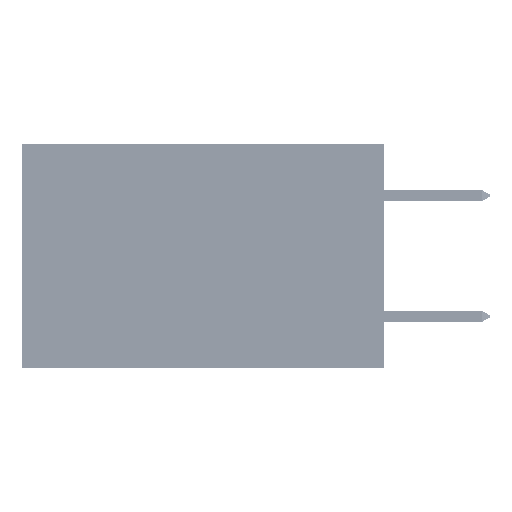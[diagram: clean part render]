
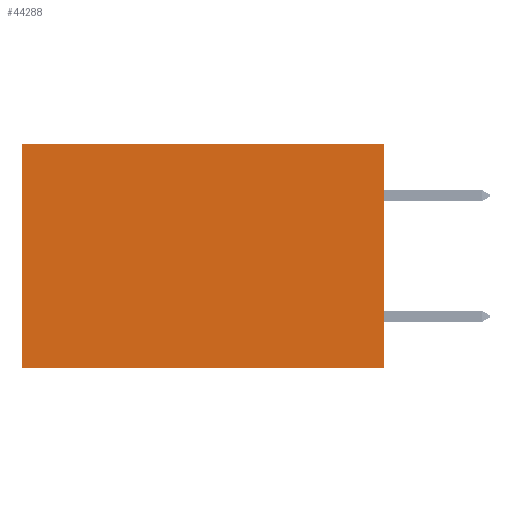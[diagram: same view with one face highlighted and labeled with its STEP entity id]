
A CAD part, left-side view. The second image highlights one B-rep face of the part: STEP entity #44288.
In plain terms, the highlighted planar face has unit normal (-1, 0, 0).
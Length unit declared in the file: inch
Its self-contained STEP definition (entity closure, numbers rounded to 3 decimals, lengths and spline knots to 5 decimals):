
#1999 = CARTESIAN_POINT ( 'NONE',  ( 0.2875, 0., 0. ) ) ;
#2432 = ORIENTED_EDGE ( 'NONE', *, *, #26261, .F. ) ;
#3375 = CARTESIAN_POINT ( 'NONE',  ( 0.2875, 0., -0.37 ) ) ;
#5676 = CARTESIAN_POINT ( 'NONE',  ( 0.2875, 0., 0. ) ) ;
#6290 = EDGE_LOOP ( 'NONE', ( #28911, #17795, #2432, #31878 ) ) ;
#8955 = CARTESIAN_POINT ( 'NONE',  ( 0.2875, 0., 0. ) ) ;
#9525 = DIRECTION ( 'NONE',  ( 0., 1., 0. ) ) ;
#9595 = PLANE ( 'NONE',  #40145 ) ;
#11863 = VECTOR ( 'NONE', #9525, 39.37008 ) ;
#17795 = ORIENTED_EDGE ( 'NONE', *, *, #31274, .F. ) ;
#17911 = DIRECTION ( 'NONE',  ( 0., 0., -1. ) ) ;
#19109 = VERTEX_POINT ( 'NONE', #43107 ) ;
#19327 = CARTESIAN_POINT ( 'NONE',  ( 0.2875, 0.6, -0.37 ) ) ;
#23286 = LINE ( 'NONE', #3375, #30376 ) ;
#25293 = DIRECTION ( 'NONE',  ( 0., 1., 0. ) ) ;
#26261 = EDGE_CURVE ( 'NONE', #33278, #19109, #46434, .T. ) ;
#26649 = DIRECTION ( 'NONE',  ( 0., 0., -1. ) ) ;
#28791 = EDGE_CURVE ( 'NONE', #33278, #43486, #31813, .T. ) ;
#28911 = ORIENTED_EDGE ( 'NONE', *, *, #46445, .T. ) ;
#30376 = VECTOR ( 'NONE', #25293, 39.37008 ) ;
#31274 = EDGE_CURVE ( 'NONE', #19109, #36460, #23286, .T. ) ;
#31813 = LINE ( 'NONE', #1999, #11863 ) ;
#31839 = VECTOR ( 'NONE', #46850, 39.37008 ) ;
#31878 = ORIENTED_EDGE ( 'NONE', *, *, #28791, .T. ) ;
#33223 = VECTOR ( 'NONE', #26649, 39.37008 ) ;
#33278 = VERTEX_POINT ( 'NONE', #46120 ) ;
#35097 = DIRECTION ( 'NONE',  ( 1., 0., 0. ) ) ;
#35324 = CARTESIAN_POINT ( 'NONE',  ( 0.2875, 0.6, 0. ) ) ;
#36460 = VERTEX_POINT ( 'NONE', #19327 ) ;
#37981 = FACE_OUTER_BOUND ( 'NONE', #6290, .T. ) ;
#38398 = LINE ( 'NONE', #45406, #33223 ) ;
#40145 = AXIS2_PLACEMENT_3D ( 'NONE', #8955, #35097, #17911 ) ;
#43107 = CARTESIAN_POINT ( 'NONE',  ( 0.2875, 0., -0.37 ) ) ;
#43486 = VERTEX_POINT ( 'NONE', #35324 ) ;
#44288 = ADVANCED_FACE ( 'NONE', ( #37981 ), #9595, .F. ) ;
#45406 = CARTESIAN_POINT ( 'NONE',  ( 0.2875, 0.6, 0. ) ) ;
#46120 = CARTESIAN_POINT ( 'NONE',  ( 0.2875, 0., 0. ) ) ;
#46434 = LINE ( 'NONE', #5676, #31839 ) ;
#46445 = EDGE_CURVE ( 'NONE', #43486, #36460, #38398, .T. ) ;
#46850 = DIRECTION ( 'NONE',  ( 0., 0., -1. ) ) ;
